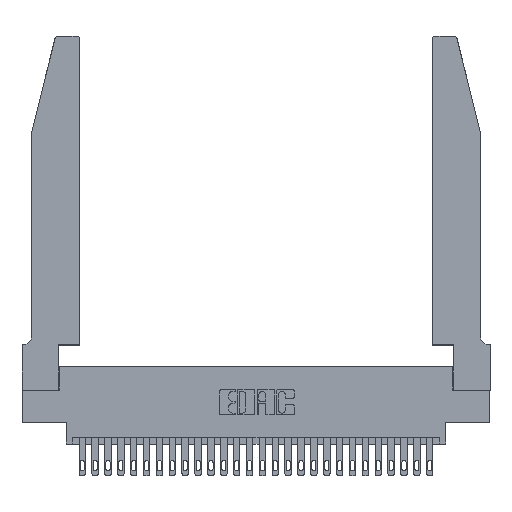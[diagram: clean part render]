
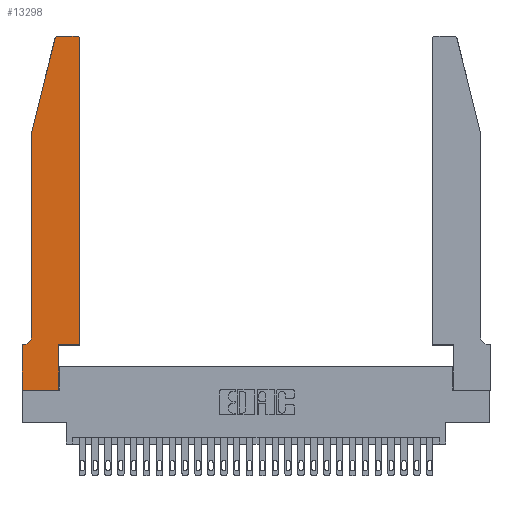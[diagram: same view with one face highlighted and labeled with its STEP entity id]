
A CAD part, top view. The second image highlights one B-rep face of the part: STEP entity #13298.
In plain terms, the highlighted planar face has unit normal (0, 0, 1).
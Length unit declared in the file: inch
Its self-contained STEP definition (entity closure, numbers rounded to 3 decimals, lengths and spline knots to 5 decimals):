
#537 = CARTESIAN_POINT ( 'NONE',  ( 0.4505, 2.72, 0.37 ) ) ;
#956 = EDGE_LOOP ( 'NONE', ( #26820, #4690, #24440, #5159, #27281, #13453, #12947, #16601, #5020, #21249, #7119, #18391 ) ) ;
#1088 = CIRCLE ( 'NONE', #25645, 0.03 ) ;
#1801 = CARTESIAN_POINT ( 'NONE',  ( 0.0055, 0.42, 0.37 ) ) ;
#2395 = AXIS2_PLACEMENT_3D ( 'NONE', #19010, #7649, #3259 ) ;
#2449 = VERTEX_POINT ( 'NONE', #19771 ) ;
#2698 = EDGE_CURVE ( 'NONE', #27696, #11774, #8987, .T. ) ;
#2895 = CARTESIAN_POINT ( 'NONE',  ( 0.2605, 2.75, 0.37 ) ) ;
#3249 = VERTEX_POINT ( 'NONE', #8435 ) ;
#3259 = DIRECTION ( 'NONE',  ( 1., 0., 0. ) ) ;
#3348 = PLANE ( 'NONE',  #12800 ) ;
#4656 = CARTESIAN_POINT ( 'NONE',  ( 0.4205, 2.75, 0.37 ) ) ;
#4690 = ORIENTED_EDGE ( 'NONE', *, *, #17304, .T. ) ;
#4700 = DIRECTION ( 'NONE',  ( 0., 1., 0. ) ) ;
#5020 = ORIENTED_EDGE ( 'NONE', *, *, #8567, .T. ) ;
#5159 = ORIENTED_EDGE ( 'NONE', *, *, #22814, .T. ) ;
#5464 = DIRECTION ( 'NONE',  ( -1., 0., 0. ) ) ;
#5587 = DIRECTION ( 'NONE',  ( 0., 0., 1. ) ) ;
#5932 = LINE ( 'NONE', #6356, #23163 ) ;
#6308 = CIRCLE ( 'NONE', #2395, 0.03 ) ;
#6348 = VECTOR ( 'NONE', #10590, 39.37008 ) ;
#6356 = CARTESIAN_POINT ( 'NONE',  ( 0., 0., 0.37 ) ) ;
#6563 = CIRCLE ( 'NONE', #16493, 0.07 ) ;
#6941 = CARTESIAN_POINT ( 'NONE',  ( 0.0755, 2., 0.37 ) ) ;
#7119 = ORIENTED_EDGE ( 'NONE', *, *, #27863, .T. ) ;
#7238 = CARTESIAN_POINT ( 'NONE',  ( 0.0055, 0.35, 0.37 ) ) ;
#7312 = VERTEX_POINT ( 'NONE', #16096 ) ;
#7435 = DIRECTION ( 'NONE',  ( -1., 0., 0. ) ) ;
#7649 = DIRECTION ( 'NONE',  ( 0., 0., 1. ) ) ;
#8023 = DIRECTION ( 'NONE',  ( 1., 0., 0. ) ) ;
#8233 = CARTESIAN_POINT ( 'NONE',  ( 0.284, 2.72, 0.37 ) ) ;
#8435 = CARTESIAN_POINT ( 'NONE',  ( 0.4505, 0.35, 0.37 ) ) ;
#8547 = EDGE_CURVE ( 'NONE', #12911, #9277, #6308, .T. ) ;
#8567 = EDGE_CURVE ( 'NONE', #21420, #25275, #20066, .T. ) ;
#8850 = FACE_OUTER_BOUND ( 'NONE', #956, .T. ) ;
#8887 = DIRECTION ( 'NONE',  ( 0., -1., 0. ) ) ;
#8987 = LINE ( 'NONE', #22559, #15172 ) ;
#9174 = EDGE_CURVE ( 'NONE', #11774, #26630, #5932, .T. ) ;
#9277 = VERTEX_POINT ( 'NONE', #4656 ) ;
#9611 = EDGE_CURVE ( 'NONE', #13975, #27696, #6563, .T. ) ;
#10590 = DIRECTION ( 'NONE',  ( 1., 0., 0. ) ) ;
#10716 = VECTOR ( 'NONE', #8887, 39.37008 ) ;
#10915 = DIRECTION ( 'NONE',  ( 1., 0., 0. ) ) ;
#10968 = VECTOR ( 'NONE', #19108, 39.37008 ) ;
#11154 = EDGE_CURVE ( 'NONE', #26630, #21420, #18208, .T. ) ;
#11693 = CARTESIAN_POINT ( 'NONE',  ( 0., 0., 0.37 ) ) ;
#11774 = VERTEX_POINT ( 'NONE', #13869 ) ;
#12073 = DIRECTION ( 'NONE',  ( 1., 0., 0. ) ) ;
#12800 = AXIS2_PLACEMENT_3D ( 'NONE', #18818, #5587, #10915 ) ;
#12911 = VERTEX_POINT ( 'NONE', #537 ) ;
#12947 = ORIENTED_EDGE ( 'NONE', *, *, #9174, .T. ) ;
#13004 = VECTOR ( 'NONE', #21085, 39.37008 ) ;
#13298 = ADVANCED_FACE ( 'NONE', ( #8850 ), #3348, .T. ) ;
#13301 = DIRECTION ( 'NONE',  ( 0., -1., 0. ) ) ;
#13453 = ORIENTED_EDGE ( 'NONE', *, *, #2698, .T. ) ;
#13782 = VECTOR ( 'NONE', #18637, 39.37008 ) ;
#13840 = VERTEX_POINT ( 'NONE', #6941 ) ;
#13869 = CARTESIAN_POINT ( 'NONE',  ( 0., 0.35, 0.37 ) ) ;
#13975 = VERTEX_POINT ( 'NONE', #15775 ) ;
#14104 = EDGE_CURVE ( 'NONE', #7312, #13840, #16837, .T. ) ;
#14466 = DIRECTION ( 'NONE',  ( 0., 0., 1. ) ) ;
#14489 = LINE ( 'NONE', #2895, #13782 ) ;
#15172 = VECTOR ( 'NONE', #7435, 39.37008 ) ;
#15775 = CARTESIAN_POINT ( 'NONE',  ( 0.0755, 0.42, 0.37 ) ) ;
#16096 = CARTESIAN_POINT ( 'NONE',  ( 0.25487, 2.72718, 0.37 ) ) ;
#16224 = LINE ( 'NONE', #26557, #10716 ) ;
#16493 = AXIS2_PLACEMENT_3D ( 'NONE', #1801, #21697, #5464 ) ;
#16601 = ORIENTED_EDGE ( 'NONE', *, *, #11154, .T. ) ;
#16672 = CARTESIAN_POINT ( 'NONE',  ( 0.4505, 0.35, 0.37 ) ) ;
#16837 = LINE ( 'NONE', #16911, #10968 ) ;
#16911 = CARTESIAN_POINT ( 'NONE',  ( 0.0755, 2., 0.37 ) ) ;
#17304 = EDGE_CURVE ( 'NONE', #2449, #7312, #1088, .T. ) ;
#18208 = LINE ( 'NONE', #11693, #25145 ) ;
#18337 = CARTESIAN_POINT ( 'NONE',  ( 0.2865, 0.35, 0.37 ) ) ;
#18391 = ORIENTED_EDGE ( 'NONE', *, *, #8547, .T. ) ;
#18536 = LINE ( 'NONE', #16672, #13004 ) ;
#18595 = CARTESIAN_POINT ( 'NONE',  ( 0.2865, 0., 0.37 ) ) ;
#18637 = DIRECTION ( 'NONE',  ( -1., 0., 0. ) ) ;
#18818 = CARTESIAN_POINT ( 'NONE',  ( 0., 0.35, 0.37 ) ) ;
#19010 = CARTESIAN_POINT ( 'NONE',  ( 0.4205, 2.72, 0.37 ) ) ;
#19108 = DIRECTION ( 'NONE',  ( -0.239, -0.971, 0. ) ) ;
#19433 = EDGE_CURVE ( 'NONE', #9277, #2449, #14489, .T. ) ;
#19771 = CARTESIAN_POINT ( 'NONE',  ( 0.284, 2.75, 0.37 ) ) ;
#20066 = LINE ( 'NONE', #18337, #23900 ) ;
#21085 = DIRECTION ( 'NONE',  ( 0., 1., 0. ) ) ;
#21249 = ORIENTED_EDGE ( 'NONE', *, *, #23429, .T. ) ;
#21420 = VERTEX_POINT ( 'NONE', #18595 ) ;
#21697 = DIRECTION ( 'NONE',  ( 0., 0., -1. ) ) ;
#22189 = LINE ( 'NONE', #28377, #6348 ) ;
#22353 = CARTESIAN_POINT ( 'NONE',  ( 0.2865, 0.35, 0.37 ) ) ;
#22559 = CARTESIAN_POINT ( 'NONE',  ( 0.0755, 0.35, 0.37 ) ) ;
#22814 = EDGE_CURVE ( 'NONE', #13840, #13975, #16224, .T. ) ;
#23163 = VECTOR ( 'NONE', #13301, 39.37008 ) ;
#23429 = EDGE_CURVE ( 'NONE', #25275, #3249, #22189, .T. ) ;
#23900 = VECTOR ( 'NONE', #4700, 39.37008 ) ;
#24440 = ORIENTED_EDGE ( 'NONE', *, *, #14104, .T. ) ;
#25145 = VECTOR ( 'NONE', #12073, 39.37008 ) ;
#25275 = VERTEX_POINT ( 'NONE', #22353 ) ;
#25645 = AXIS2_PLACEMENT_3D ( 'NONE', #8233, #14466, #8023 ) ;
#26557 = CARTESIAN_POINT ( 'NONE',  ( 0.0755, 2., 0.37 ) ) ;
#26630 = VERTEX_POINT ( 'NONE', #28374 ) ;
#26820 = ORIENTED_EDGE ( 'NONE', *, *, #19433, .T. ) ;
#27281 = ORIENTED_EDGE ( 'NONE', *, *, #9611, .T. ) ;
#27696 = VERTEX_POINT ( 'NONE', #7238 ) ;
#27863 = EDGE_CURVE ( 'NONE', #3249, #12911, #18536, .T. ) ;
#28374 = CARTESIAN_POINT ( 'NONE',  ( 0., 0., 0.37 ) ) ;
#28377 = CARTESIAN_POINT ( 'NONE',  ( 0.4505, 0.35, 0.37 ) ) ;
